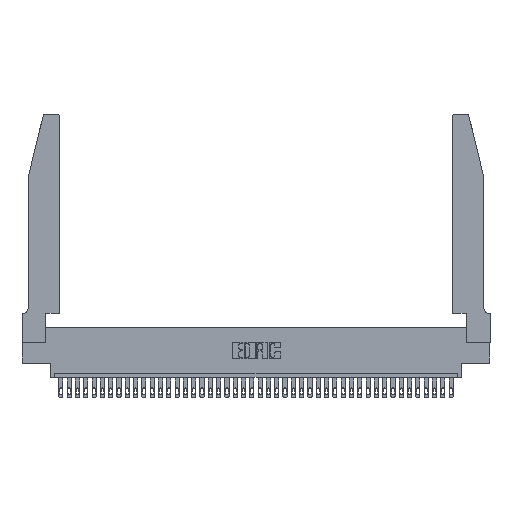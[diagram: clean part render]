
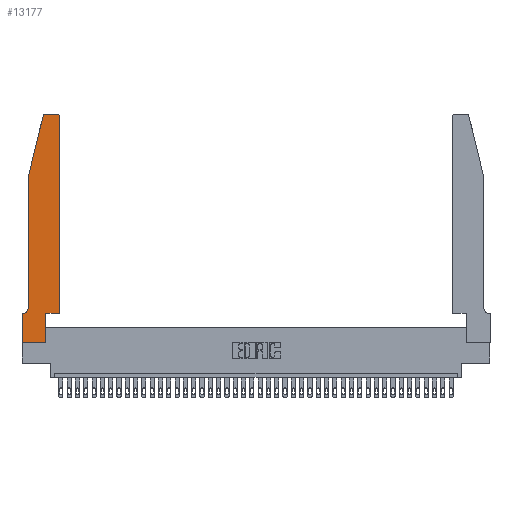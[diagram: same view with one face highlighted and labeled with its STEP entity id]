
A CAD part, top view. The second image highlights one B-rep face of the part: STEP entity #13177.
In plain terms, the highlighted planar face has unit normal (0, 0, 1).
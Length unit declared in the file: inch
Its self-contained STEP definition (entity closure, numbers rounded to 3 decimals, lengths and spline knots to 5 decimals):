
#564 = LINE ( 'NONE', #10087, #29723 ) ;
#877 = ORIENTED_EDGE ( 'NONE', *, *, #6304, .T. ) ;
#1187 = CARTESIAN_POINT ( 'NONE',  ( 0.284, 2.72, 0.37 ) ) ;
#1223 = CARTESIAN_POINT ( 'NONE',  ( 0.4505, 0.35, 0.37 ) ) ;
#1365 = DIRECTION ( 'NONE',  ( 1., 0., 0. ) ) ;
#1952 = CARTESIAN_POINT ( 'NONE',  ( 0.25487, 2.72718, 0.37 ) ) ;
#1962 = VERTEX_POINT ( 'NONE', #24189 ) ;
#2208 = LINE ( 'NONE', #8422, #19595 ) ;
#2367 = VECTOR ( 'NONE', #1365, 39.37008 ) ;
#3619 = DIRECTION ( 'NONE',  ( -1., 0., 0. ) ) ;
#5104 = VECTOR ( 'NONE', #10131, 39.37008 ) ;
#5628 = VERTEX_POINT ( 'NONE', #15203 ) ;
#5961 = LINE ( 'NONE', #21606, #20520 ) ;
#5985 = DIRECTION ( 'NONE',  ( 1., 0., 0. ) ) ;
#6088 = DIRECTION ( 'NONE',  ( 0., 1., 0. ) ) ;
#6304 = EDGE_CURVE ( 'NONE', #38870, #37118, #11844, .T. ) ;
#6310 = CARTESIAN_POINT ( 'NONE',  ( 0.0755, 2., 0.37 ) ) ;
#6504 = EDGE_CURVE ( 'NONE', #1962, #38870, #17185, .T. ) ;
#6976 = VERTEX_POINT ( 'NONE', #22828 ) ;
#7261 = DIRECTION ( 'NONE',  ( 1., 0., 0. ) ) ;
#7543 = VERTEX_POINT ( 'NONE', #33934 ) ;
#7612 = AXIS2_PLACEMENT_3D ( 'NONE', #1187, #19859, #7261 ) ;
#7903 = DIRECTION ( 'NONE',  ( -1., 0., 0. ) ) ;
#7999 = LINE ( 'NONE', #32588, #33787 ) ;
#8043 = VECTOR ( 'NONE', #22725, 39.37008 ) ;
#8422 = CARTESIAN_POINT ( 'NONE',  ( 0., 0., 0.37 ) ) ;
#8683 = VERTEX_POINT ( 'NONE', #25953 ) ;
#9231 = VECTOR ( 'NONE', #6088, 39.37008 ) ;
#9250 = EDGE_CURVE ( 'NONE', #6976, #37993, #15025, .T. ) ;
#9675 = VERTEX_POINT ( 'NONE', #15429 ) ;
#10087 = CARTESIAN_POINT ( 'NONE',  ( 0.2605, 2.75, 0.37 ) ) ;
#10131 = DIRECTION ( 'NONE',  ( 0., 1., 0. ) ) ;
#10672 = DIRECTION ( 'NONE',  ( 1., 0., 0. ) ) ;
#11053 = LINE ( 'NONE', #1223, #2367 ) ;
#11653 = ORIENTED_EDGE ( 'NONE', *, *, #6504, .T. ) ;
#11728 = ORIENTED_EDGE ( 'NONE', *, *, #9250, .T. ) ;
#11844 = LINE ( 'NONE', #19597, #8043 ) ;
#13133 = FACE_OUTER_BOUND ( 'NONE', #36810, .T. ) ;
#13177 = ADVANCED_FACE ( 'NONE', ( #13133 ), #27775, .T. ) ;
#13651 = ORIENTED_EDGE ( 'NONE', *, *, #20761, .T. ) ;
#14536 = EDGE_CURVE ( 'NONE', #8683, #33922, #34155, .T. ) ;
#15025 = CIRCLE ( 'NONE', #15877, 0.07 ) ;
#15203 = CARTESIAN_POINT ( 'NONE',  ( 0., 0., 0.37 ) ) ;
#15429 = CARTESIAN_POINT ( 'NONE',  ( 0.2865, 0., 0.37 ) ) ;
#15554 = VECTOR ( 'NONE', #23322, 39.37008 ) ;
#15757 = EDGE_CURVE ( 'NONE', #23073, #1962, #564, .T. ) ;
#15877 = AXIS2_PLACEMENT_3D ( 'NONE', #20488, #23323, #7903 ) ;
#15979 = CARTESIAN_POINT ( 'NONE',  ( 0.0055, 0.35, 0.37 ) ) ;
#16465 = LINE ( 'NONE', #25752, #9231 ) ;
#16928 = ORIENTED_EDGE ( 'NONE', *, *, #25845, .T. ) ;
#17185 = CIRCLE ( 'NONE', #7612, 0.03 ) ;
#19595 = VECTOR ( 'NONE', #30103, 39.37008 ) ;
#19597 = CARTESIAN_POINT ( 'NONE',  ( 0.0755, 2., 0.37 ) ) ;
#19859 = DIRECTION ( 'NONE',  ( 0., 0., 1. ) ) ;
#19938 = ORIENTED_EDGE ( 'NONE', *, *, #35100, .T. ) ;
#20357 = CARTESIAN_POINT ( 'NONE',  ( 0., 0., 0.37 ) ) ;
#20488 = CARTESIAN_POINT ( 'NONE',  ( 0.0055, 0.42, 0.37 ) ) ;
#20520 = VECTOR ( 'NONE', #24720, 39.37008 ) ;
#20761 = EDGE_CURVE ( 'NONE', #33922, #23073, #37407, .T. ) ;
#21079 = EDGE_CURVE ( 'NONE', #9675, #7543, #16465, .T. ) ;
#21490 = CARTESIAN_POINT ( 'NONE',  ( 0.4205, 2.75, 0.37 ) ) ;
#21606 = CARTESIAN_POINT ( 'NONE',  ( 0.0755, 0.35, 0.37 ) ) ;
#22725 = DIRECTION ( 'NONE',  ( -0.239, -0.971, 0. ) ) ;
#22828 = CARTESIAN_POINT ( 'NONE',  ( 0.0755, 0.42, 0.37 ) ) ;
#23073 = VERTEX_POINT ( 'NONE', #21490 ) ;
#23279 = CARTESIAN_POINT ( 'NONE',  ( 0.4205, 2.72, 0.37 ) ) ;
#23322 = DIRECTION ( 'NONE',  ( 1., 0., 0. ) ) ;
#23323 = DIRECTION ( 'NONE',  ( 0., 0., -1. ) ) ;
#23350 = ORIENTED_EDGE ( 'NONE', *, *, #36309, .T. ) ;
#24189 = CARTESIAN_POINT ( 'NONE',  ( 0.284, 2.75, 0.37 ) ) ;
#24720 = DIRECTION ( 'NONE',  ( -1., 0., 0. ) ) ;
#25731 = VERTEX_POINT ( 'NONE', #34315 ) ;
#25752 = CARTESIAN_POINT ( 'NONE',  ( 0.2865, 0.35, 0.37 ) ) ;
#25845 = EDGE_CURVE ( 'NONE', #37118, #6976, #7999, .T. ) ;
#25953 = CARTESIAN_POINT ( 'NONE',  ( 0.4505, 0.35, 0.37 ) ) ;
#26114 = DIRECTION ( 'NONE',  ( 0., 0., 1. ) ) ;
#27775 = PLANE ( 'NONE',  #33506 ) ;
#28373 = EDGE_CURVE ( 'NONE', #7543, #8683, #11053, .T. ) ;
#28712 = CARTESIAN_POINT ( 'NONE',  ( 0.4505, 0.35, 0.37 ) ) ;
#29230 = LINE ( 'NONE', #20357, #15554 ) ;
#29469 = ORIENTED_EDGE ( 'NONE', *, *, #21079, .T. ) ;
#29692 = ORIENTED_EDGE ( 'NONE', *, *, #30084, .T. ) ;
#29723 = VECTOR ( 'NONE', #3619, 39.37008 ) ;
#30084 = EDGE_CURVE ( 'NONE', #25731, #5628, #2208, .T. ) ;
#30103 = DIRECTION ( 'NONE',  ( 0., -1., 0. ) ) ;
#32588 = CARTESIAN_POINT ( 'NONE',  ( 0.0755, 2., 0.37 ) ) ;
#33506 = AXIS2_PLACEMENT_3D ( 'NONE', #37048, #40134, #5985 ) ;
#33787 = VECTOR ( 'NONE', #38842, 39.37008 ) ;
#33922 = VERTEX_POINT ( 'NONE', #35950 ) ;
#33934 = CARTESIAN_POINT ( 'NONE',  ( 0.2865, 0.35, 0.37 ) ) ;
#34155 = LINE ( 'NONE', #28712, #5104 ) ;
#34315 = CARTESIAN_POINT ( 'NONE',  ( 0., 0.35, 0.37 ) ) ;
#35100 = EDGE_CURVE ( 'NONE', #37993, #25731, #5961, .T. ) ;
#35845 = ORIENTED_EDGE ( 'NONE', *, *, #28373, .T. ) ;
#35950 = CARTESIAN_POINT ( 'NONE',  ( 0.4505, 2.72, 0.37 ) ) ;
#36284 = ORIENTED_EDGE ( 'NONE', *, *, #15757, .T. ) ;
#36309 = EDGE_CURVE ( 'NONE', #5628, #9675, #29230, .T. ) ;
#36810 = EDGE_LOOP ( 'NONE', ( #36284, #11653, #877, #16928, #11728, #19938, #29692, #23350, #29469, #35845, #37242, #13651 ) ) ;
#37048 = CARTESIAN_POINT ( 'NONE',  ( 0., 0.35, 0.37 ) ) ;
#37118 = VERTEX_POINT ( 'NONE', #6310 ) ;
#37242 = ORIENTED_EDGE ( 'NONE', *, *, #14536, .T. ) ;
#37407 = CIRCLE ( 'NONE', #38117, 0.03 ) ;
#37993 = VERTEX_POINT ( 'NONE', #15979 ) ;
#38117 = AXIS2_PLACEMENT_3D ( 'NONE', #23279, #26114, #10672 ) ;
#38842 = DIRECTION ( 'NONE',  ( 0., -1., 0. ) ) ;
#38870 = VERTEX_POINT ( 'NONE', #1952 ) ;
#40134 = DIRECTION ( 'NONE',  ( 0., 0., 1. ) ) ;
